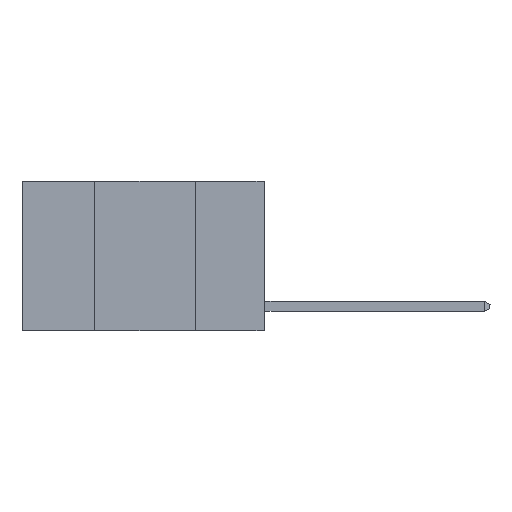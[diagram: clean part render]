
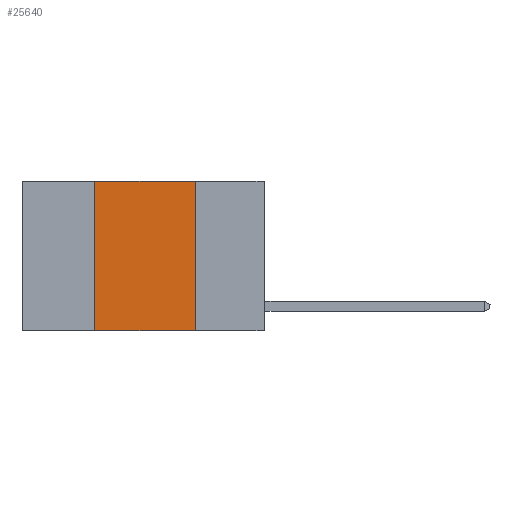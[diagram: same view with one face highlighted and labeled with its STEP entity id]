
A CAD part, left-side view. The second image highlights one B-rep face of the part: STEP entity #25640.
In plain terms, the highlighted planar face has unit normal (-1, 0, 0).
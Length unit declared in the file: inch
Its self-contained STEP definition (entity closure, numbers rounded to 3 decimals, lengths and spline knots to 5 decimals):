
#765 = CARTESIAN_POINT ( 'NONE',  ( 0., 0.42, -0.37 ) ) ;
#1321 = DIRECTION ( 'NONE',  ( 0., -1., 0. ) ) ;
#1941 = CARTESIAN_POINT ( 'NONE',  ( 0., 0.6, 0. ) ) ;
#2057 = LINE ( 'NONE', #7495, #13638 ) ;
#2790 = EDGE_CURVE ( 'NONE', #29428, #11853, #2057, .T. ) ;
#2972 = CARTESIAN_POINT ( 'NONE',  ( 0., 0.6, -0.37 ) ) ;
#3352 = ORIENTED_EDGE ( 'NONE', *, *, #21378, .F. ) ;
#4717 = LINE ( 'NONE', #10494, #10846 ) ;
#4793 = ORIENTED_EDGE ( 'NONE', *, *, #2790, .F. ) ;
#5041 = LINE ( 'NONE', #29048, #10417 ) ;
#5292 = DIRECTION ( 'NONE',  ( 0., -1., 0. ) ) ;
#5445 = FACE_OUTER_BOUND ( 'NONE', #17380, .T. ) ;
#5489 = CARTESIAN_POINT ( 'NONE',  ( 0., 0.17, -0.37 ) ) ;
#6276 = VERTEX_POINT ( 'NONE', #11156 ) ;
#7495 = CARTESIAN_POINT ( 'NONE',  ( 0., 0.42, 0. ) ) ;
#8890 = PLANE ( 'NONE',  #22759 ) ;
#9345 = VERTEX_POINT ( 'NONE', #5489 ) ;
#10417 = VECTOR ( 'NONE', #24496, 39.37008 ) ;
#10494 = CARTESIAN_POINT ( 'NONE',  ( 0., 0.6, 0. ) ) ;
#10846 = VECTOR ( 'NONE', #1321, 39.37008 ) ;
#11156 = CARTESIAN_POINT ( 'NONE',  ( 0., 0.17, 0. ) ) ;
#11217 = DIRECTION ( 'NONE',  ( 1., 0., 0. ) ) ;
#11853 = VERTEX_POINT ( 'NONE', #18633 ) ;
#12219 = EDGE_CURVE ( 'NONE', #11853, #6276, #4717, .T. ) ;
#12724 = LINE ( 'NONE', #2972, #24323 ) ;
#13638 = VECTOR ( 'NONE', #26033, 39.37008 ) ;
#16369 = ORIENTED_EDGE ( 'NONE', *, *, #12219, .F. ) ;
#17380 = EDGE_LOOP ( 'NONE', ( #3352, #16369, #4793, #17821 ) ) ;
#17821 = ORIENTED_EDGE ( 'NONE', *, *, #18854, .T. ) ;
#18633 = CARTESIAN_POINT ( 'NONE',  ( 0., 0.42, 0. ) ) ;
#18854 = EDGE_CURVE ( 'NONE', #29428, #9345, #12724, .T. ) ;
#21378 = EDGE_CURVE ( 'NONE', #6276, #9345, #5041, .T. ) ;
#22759 = AXIS2_PLACEMENT_3D ( 'NONE', #1941, #11217, #27393 ) ;
#24323 = VECTOR ( 'NONE', #5292, 39.37008 ) ;
#24496 = DIRECTION ( 'NONE',  ( 0., 0., -1. ) ) ;
#25640 = ADVANCED_FACE ( 'NONE', ( #5445 ), #8890, .F. ) ;
#26033 = DIRECTION ( 'NONE',  ( 0., 0., 1. ) ) ;
#27393 = DIRECTION ( 'NONE',  ( 0., 0., -1. ) ) ;
#29048 = CARTESIAN_POINT ( 'NONE',  ( 0., 0.17, 0. ) ) ;
#29428 = VERTEX_POINT ( 'NONE', #765 ) ;
